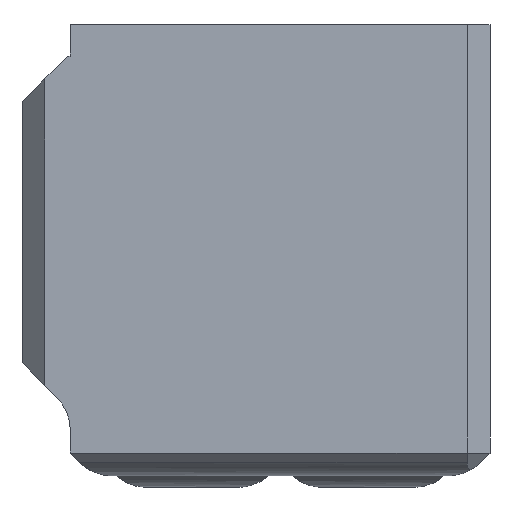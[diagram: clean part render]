
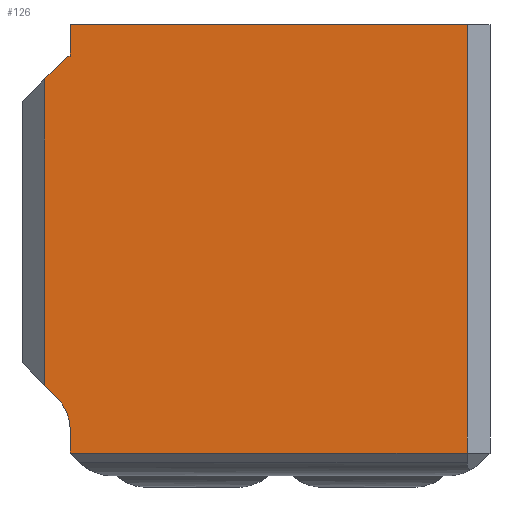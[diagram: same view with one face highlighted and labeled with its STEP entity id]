
A CAD part, front view. The second image highlights one B-rep face of the part: STEP entity #126.
In plain terms, the highlighted planar face has unit normal (0, -1, 0).
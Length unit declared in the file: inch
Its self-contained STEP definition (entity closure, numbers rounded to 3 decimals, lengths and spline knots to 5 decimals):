
#9 = EDGE_CURVE ( 'NONE', #227, #233, #1032, .T. ) ;
#34 = EDGE_CURVE ( 'NONE', #250, #241, #1076, .T. ) ;
#38 = EDGE_CURVE ( 'NONE', #233, #250, #139, .T. ) ;
#42 = EDGE_CURVE ( 'NONE', #207, #218, #805, .T. ) ;
#45 = EDGE_CURVE ( 'NONE', #201, #200, #823, .T. ) ;
#51 = EDGE_CURVE ( 'NONE', #201, #218, #836, .T. ) ;
#55 = EDGE_CURVE ( 'NONE', #251, #227, #841, .T. ) ;
#56 = EDGE_CURVE ( 'NONE', #207, #251, #855, .T. ) ;
#57 = EDGE_CURVE ( 'NONE', #241, #252, #837, .T. ) ;
#62 = EDGE_CURVE ( 'NONE', #252, #200, #862, .T. ) ;
#126 = ADVANCED_FACE ( 'NONE', ( #402 ), #468, .F. ) ;
#139 = CIRCLE ( 'NONE', #273, 0.3937 ) ;
#156 = ORIENTED_EDGE ( 'NONE', *, *, #34, .T. ) ;
#159 = ORIENTED_EDGE ( 'NONE', *, *, #62, .T. ) ;
#161 = ORIENTED_EDGE ( 'NONE', *, *, #57, .T. ) ;
#166 = ORIENTED_EDGE ( 'NONE', *, *, #42, .F. ) ;
#171 = ORIENTED_EDGE ( 'NONE', *, *, #38, .T. ) ;
#177 = ORIENTED_EDGE ( 'NONE', *, *, #9, .T. ) ;
#180 = ORIENTED_EDGE ( 'NONE', *, *, #51, .T. ) ;
#182 = ORIENTED_EDGE ( 'NONE', *, *, #45, .F. ) ;
#200 = VERTEX_POINT ( 'NONE', #643 ) ;
#201 = VERTEX_POINT ( 'NONE', #636 ) ;
#207 = VERTEX_POINT ( 'NONE', #648 ) ;
#218 = VERTEX_POINT ( 'NONE', #637 ) ;
#227 = VERTEX_POINT ( 'NONE', #656 ) ;
#233 = VERTEX_POINT ( 'NONE', #690 ) ;
#241 = VERTEX_POINT ( 'NONE', #696 ) ;
#250 = VERTEX_POINT ( 'NONE', #670 ) ;
#251 = VERTEX_POINT ( 'NONE', #677 ) ;
#252 = VERTEX_POINT ( 'NONE', #672 ) ;
#266 = VECTOR ( 'NONE', #1039, 39.37008 ) ;
#273 = AXIS2_PLACEMENT_3D ( 'NONE', #1134, #1072, #1078 ) ;
#300 = VECTOR ( 'NONE', #811, 39.37008 ) ;
#301 = VECTOR ( 'NONE', #812, 39.37008 ) ;
#303 = VECTOR ( 'NONE', #1070, 39.37008 ) ;
#306 = VECTOR ( 'NONE', #840, 39.37008 ) ;
#307 = VECTOR ( 'NONE', #829, 39.37008 ) ;
#310 = VECTOR ( 'NONE', #827, 39.37008 ) ;
#312 = VECTOR ( 'NONE', #864, 39.37008 ) ;
#313 = VECTOR ( 'NONE', #847, 39.37008 ) ;
#387 = AXIS2_PLACEMENT_3D ( 'NONE', #480, #485, #486 ) ;
#402 = FACE_OUTER_BOUND ( 'NONE', #1151, .T. ) ;
#468 = PLANE ( 'NONE',  #387 ) ;
#480 = CARTESIAN_POINT ( 'NONE',  ( 0., 0., 0. ) ) ;
#485 = DIRECTION ( 'NONE',  ( 0., 1., 0. ) ) ;
#486 = DIRECTION ( 'NONE',  ( 0., 0., 1. ) ) ;
#636 = CARTESIAN_POINT ( 'NONE',  ( 0., 0., 0. ) ) ;
#637 = CARTESIAN_POINT ( 'NONE',  ( 0., 0., -0.27148 ) ) ;
#643 = CARTESIAN_POINT ( 'NONE',  ( 3.42315, 0., 0. ) ) ;
#648 = CARTESIAN_POINT ( 'NONE',  ( -0.022, 0., -0.27148 ) ) ;
#656 = CARTESIAN_POINT ( 'NONE',  ( -0.21885, 0., -3.11274 ) ) ;
#670 = CARTESIAN_POINT ( 'NONE',  ( 0., 0., -3.49467 ) ) ;
#672 = CARTESIAN_POINT ( 'NONE',  ( 3.42315, 0., -3.69471 ) ) ;
#677 = CARTESIAN_POINT ( 'NONE',  ( -0.21885, 0., -0.46833 ) ) ;
#690 = CARTESIAN_POINT ( 'NONE',  ( -0.11531, 0., -3.21628 ) ) ;
#696 = CARTESIAN_POINT ( 'NONE',  ( 0., 0., -3.69471 ) ) ;
#795 = CARTESIAN_POINT ( 'NONE',  ( 0., 0., -0.27148 ) ) ;
#805 = LINE ( 'NONE', #795, #300 ) ;
#811 = DIRECTION ( 'NONE',  ( 1., 0., 0. ) ) ;
#812 = DIRECTION ( 'NONE',  ( 1., 0., 0. ) ) ;
#823 = LINE ( 'NONE', #824, #301 ) ;
#824 = CARTESIAN_POINT ( 'NONE',  ( 0., 0., 0. ) ) ;
#827 = DIRECTION ( 'NONE',  ( 0., 0., -1. ) ) ;
#829 = DIRECTION ( 'NONE',  ( -0.707, 0., -0.707 ) ) ;
#833 = CARTESIAN_POINT ( 'NONE',  ( -0.21885, 0., 0. ) ) ;
#836 = LINE ( 'NONE', #839, #310 ) ;
#837 = LINE ( 'NONE', #846, #313 ) ;
#839 = CARTESIAN_POINT ( 'NONE',  ( 0., 0., 0. ) ) ;
#840 = DIRECTION ( 'NONE',  ( 0., 0., -1. ) ) ;
#841 = LINE ( 'NONE', #833, #306 ) ;
#846 = CARTESIAN_POINT ( 'NONE',  ( 3.62, 0., -3.69471 ) ) ;
#847 = DIRECTION ( 'NONE',  ( 1., 0., 0. ) ) ;
#851 = CARTESIAN_POINT ( 'NONE',  ( -0.022, 0., -0.27148 ) ) ;
#855 = LINE ( 'NONE', #851, #307 ) ;
#858 = CARTESIAN_POINT ( 'NONE',  ( 3.42315, 0., 0. ) ) ;
#862 = LINE ( 'NONE', #858, #312 ) ;
#864 = DIRECTION ( 'NONE',  ( 0., 0., 1. ) ) ;
#1032 = LINE ( 'NONE', #1057, #266 ) ;
#1039 = DIRECTION ( 'NONE',  ( 0.707, 0., -0.707 ) ) ;
#1057 = CARTESIAN_POINT ( 'NONE',  ( -0.4157, 0., -2.91589 ) ) ;
#1070 = DIRECTION ( 'NONE',  ( 0., 0., -1. ) ) ;
#1072 = DIRECTION ( 'NONE',  ( 0., 1., 0. ) ) ;
#1076 = LINE ( 'NONE', #1082, #303 ) ;
#1078 = DIRECTION ( 'NONE',  ( 0., 0., 1. ) ) ;
#1082 = CARTESIAN_POINT ( 'NONE',  ( 0., 0., 0. ) ) ;
#1134 = CARTESIAN_POINT ( 'NONE',  ( -0.3937, 0., -3.49467 ) ) ;
#1145 = ORIENTED_EDGE ( 'NONE', *, *, #56, .T. ) ;
#1151 = EDGE_LOOP ( 'NONE', ( #177, #171, #156, #161, #159, #182, #180, #166, #1145, #1175 ) ) ;
#1175 = ORIENTED_EDGE ( 'NONE', *, *, #55, .T. ) ;
